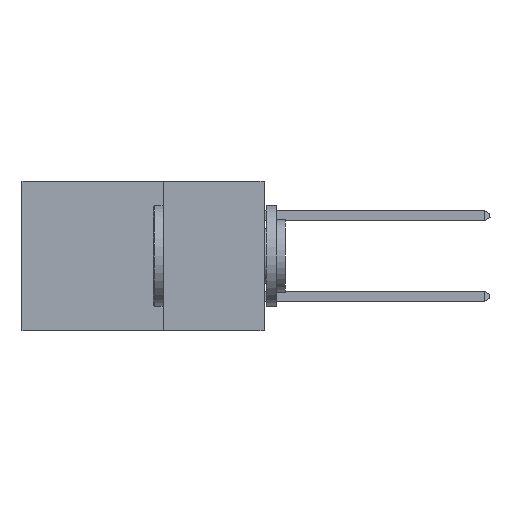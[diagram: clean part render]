
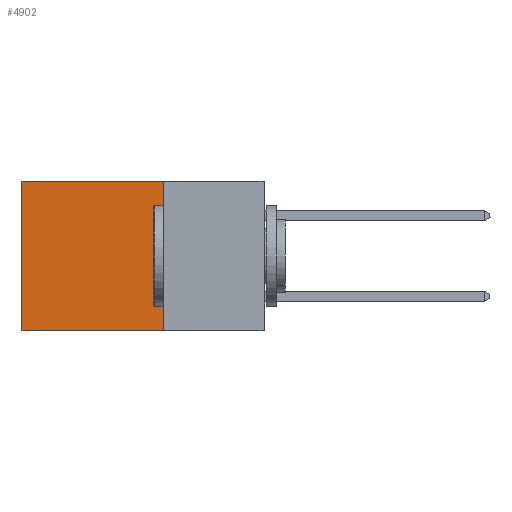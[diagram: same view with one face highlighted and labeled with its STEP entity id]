
A CAD part, left-side view. The second image highlights one B-rep face of the part: STEP entity #4902.
In plain terms, the highlighted planar face has unit normal (-1, 0, 0).
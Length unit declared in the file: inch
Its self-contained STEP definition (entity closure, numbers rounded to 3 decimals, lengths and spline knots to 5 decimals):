
#419 = CARTESIAN_POINT ( 'NONE',  ( 0.298, 0.25, 0. ) ) ;
#727 = LINE ( 'NONE', #6887, #1190 ) ;
#821 = CARTESIAN_POINT ( 'NONE',  ( 0.298, 0.25, 0. ) ) ;
#1190 = VECTOR ( 'NONE', #9063, 39.37008 ) ;
#1328 = DIRECTION ( 'NONE',  ( 1., 0., 0. ) ) ;
#1514 = AXIS2_PLACEMENT_3D ( 'NONE', #419, #1328, #9500 ) ;
#1767 = ORIENTED_EDGE ( 'NONE', *, *, #11660, .T. ) ;
#1954 = DIRECTION ( 'NONE',  ( 0., 0., -1. ) ) ;
#2054 = CARTESIAN_POINT ( 'NONE',  ( 0.298, 0.6, 0. ) ) ;
#2623 = VECTOR ( 'NONE', #1954, 39.37008 ) ;
#3430 = ORIENTED_EDGE ( 'NONE', *, *, #7139, .F. ) ;
#3604 = CARTESIAN_POINT ( 'NONE',  ( 0.298, 0.25, 0. ) ) ;
#4341 = VERTEX_POINT ( 'NONE', #11595 ) ;
#4561 = VECTOR ( 'NONE', #6766, 39.37008 ) ;
#4842 = VERTEX_POINT ( 'NONE', #821 ) ;
#4902 = ADVANCED_FACE ( 'NONE', ( #12296 ), #6393, .F. ) ;
#5016 = VECTOR ( 'NONE', #9041, 39.37008 ) ;
#6167 = CARTESIAN_POINT ( 'NONE',  ( 0.298, 0.6, -0.37 ) ) ;
#6393 = PLANE ( 'NONE',  #1514 ) ;
#6609 = VERTEX_POINT ( 'NONE', #6167 ) ;
#6766 = DIRECTION ( 'NONE',  ( 0., 0., -1. ) ) ;
#6887 = CARTESIAN_POINT ( 'NONE',  ( 0.298, 0.25, -0.37 ) ) ;
#7139 = EDGE_CURVE ( 'NONE', #4842, #4341, #7589, .T. ) ;
#7589 = LINE ( 'NONE', #3604, #4561 ) ;
#7723 = LINE ( 'NONE', #9119, #5016 ) ;
#8688 = EDGE_CURVE ( 'NONE', #4842, #12176, #7723, .T. ) ;
#8796 = CARTESIAN_POINT ( 'NONE',  ( 0.298, 0.6, 0. ) ) ;
#9041 = DIRECTION ( 'NONE',  ( 0., 1., 0. ) ) ;
#9063 = DIRECTION ( 'NONE',  ( 0., 1., 0. ) ) ;
#9119 = CARTESIAN_POINT ( 'NONE',  ( 0.298, 0.25, 0. ) ) ;
#9500 = DIRECTION ( 'NONE',  ( 0., 0., -1. ) ) ;
#10049 = ORIENTED_EDGE ( 'NONE', *, *, #8688, .T. ) ;
#10768 = ORIENTED_EDGE ( 'NONE', *, *, #12306, .F. ) ;
#11595 = CARTESIAN_POINT ( 'NONE',  ( 0.298, 0.25, -0.37 ) ) ;
#11660 = EDGE_CURVE ( 'NONE', #12176, #6609, #11686, .T. ) ;
#11686 = LINE ( 'NONE', #2054, #2623 ) ;
#11776 = EDGE_LOOP ( 'NONE', ( #1767, #10768, #3430, #10049 ) ) ;
#12176 = VERTEX_POINT ( 'NONE', #8796 ) ;
#12296 = FACE_OUTER_BOUND ( 'NONE', #11776, .T. ) ;
#12306 = EDGE_CURVE ( 'NONE', #4341, #6609, #727, .T. ) ;
